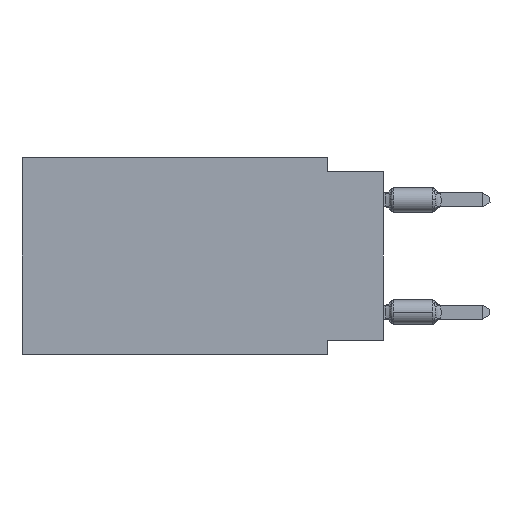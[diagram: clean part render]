
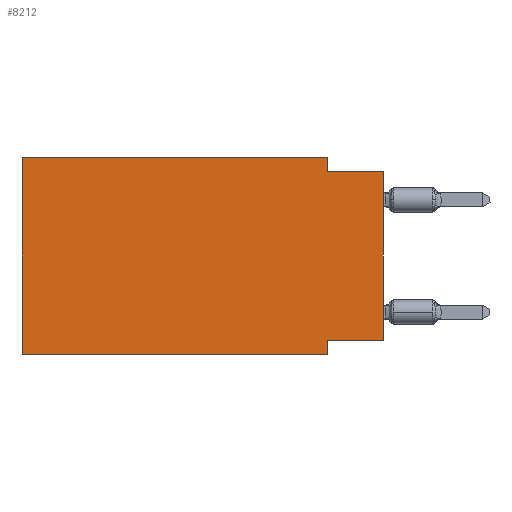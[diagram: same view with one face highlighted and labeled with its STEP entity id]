
A CAD part, left-side view. The second image highlights one B-rep face of the part: STEP entity #8212.
In plain terms, the highlighted planar face has unit normal (-1, 0, 0).
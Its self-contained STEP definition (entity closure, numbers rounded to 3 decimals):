
#36 = EDGE_CURVE ( 'NONE', #12416, #5245, #12398, .T. ) ;
#90 = DIRECTION ( 'NONE',  ( 0., -1., 0. ) ) ;
#271 = CARTESIAN_POINT ( 'NONE',  ( 0., 0., -0.635 ) ) ;
#599 = CARTESIAN_POINT ( 'NONE',  ( 0., 2.54, -0.635 ) ) ;
#840 = LINE ( 'NONE', #13821, #6699 ) ;
#1458 = DIRECTION ( 'NONE',  ( 0., -1., 0. ) ) ;
#1938 = CARTESIAN_POINT ( 'NONE',  ( 0., 0., -8.255 ) ) ;
#2111 = DIRECTION ( 'NONE',  ( 0., 1., 0. ) ) ;
#2193 = DIRECTION ( 'NONE',  ( 0., 0., 1. ) ) ;
#2235 = VERTEX_POINT ( 'NONE', #4005 ) ;
#2441 = DIRECTION ( 'NONE',  ( 0., 0., -1. ) ) ;
#2883 = ORIENTED_EDGE ( 'NONE', *, *, #16014, .F. ) ;
#3149 = CARTESIAN_POINT ( 'NONE',  ( 0., 16.383, -8.89 ) ) ;
#3205 = LINE ( 'NONE', #1938, #12406 ) ;
#3282 = VECTOR ( 'NONE', #2441, 1000. ) ;
#3781 = CARTESIAN_POINT ( 'NONE',  ( 0., 0., -8.255 ) ) ;
#3790 = EDGE_CURVE ( 'NONE', #2235, #12416, #10270, .T. ) ;
#3835 = CARTESIAN_POINT ( 'NONE',  ( 0., 2.54, -8.89 ) ) ;
#3869 = FACE_OUTER_BOUND ( 'NONE', #6715, .T. ) ;
#4005 = CARTESIAN_POINT ( 'NONE',  ( 0., 16.383, 0. ) ) ;
#4244 = CARTESIAN_POINT ( 'NONE',  ( 0., 2.54, 0. ) ) ;
#4347 = DIRECTION ( 'NONE',  ( 0., -1., 0. ) ) ;
#4388 = CARTESIAN_POINT ( 'NONE',  ( 0., 0., -0.635 ) ) ;
#5245 = VERTEX_POINT ( 'NONE', #599 ) ;
#5447 = DIRECTION ( 'NONE',  ( 0., 0., -1. ) ) ;
#5626 = LINE ( 'NONE', #3149, #8918 ) ;
#5699 = VERTEX_POINT ( 'NONE', #11560 ) ;
#6218 = VECTOR ( 'NONE', #16486, 1000. ) ;
#6660 = CARTESIAN_POINT ( 'NONE',  ( 0., 2.54, -8.255 ) ) ;
#6699 = VECTOR ( 'NONE', #2193, 1000. ) ;
#6715 = EDGE_LOOP ( 'NONE', ( #11568, #2883, #10927, #16063, #16458, #15356, #11943, #16244 ) ) ;
#7647 = EDGE_CURVE ( 'NONE', #5699, #2235, #840, .T. ) ;
#7719 = VECTOR ( 'NONE', #90, 1000. ) ;
#7919 = LINE ( 'NONE', #3835, #13597 ) ;
#8061 = AXIS2_PLACEMENT_3D ( 'NONE', #9050, #14229, #16520 ) ;
#8212 = ADVANCED_FACE ( 'NONE', ( #3869 ), #12611, .F. ) ;
#8758 = EDGE_CURVE ( 'NONE', #10169, #10735, #3205, .T. ) ;
#8918 = VECTOR ( 'NONE', #4347, 1000. ) ;
#9050 = CARTESIAN_POINT ( 'NONE',  ( 0., 16.383, 0. ) ) ;
#9596 = EDGE_CURVE ( 'NONE', #5699, #10608, #5626, .T. ) ;
#9867 = CARTESIAN_POINT ( 'NONE',  ( 0., 0., 0. ) ) ;
#10169 = VERTEX_POINT ( 'NONE', #3781 ) ;
#10270 = LINE ( 'NONE', #14008, #7719 ) ;
#10608 = VERTEX_POINT ( 'NONE', #12519 ) ;
#10735 = VERTEX_POINT ( 'NONE', #6660 ) ;
#10927 = ORIENTED_EDGE ( 'NONE', *, *, #36, .F. ) ;
#11012 = VECTOR ( 'NONE', #1458, 1000. ) ;
#11560 = CARTESIAN_POINT ( 'NONE',  ( 0., 16.383, -8.89 ) ) ;
#11568 = ORIENTED_EDGE ( 'NONE', *, *, #14661, .T. ) ;
#11943 = ORIENTED_EDGE ( 'NONE', *, *, #12275, .F. ) ;
#12275 = EDGE_CURVE ( 'NONE', #10735, #10608, #7919, .T. ) ;
#12398 = LINE ( 'NONE', #14862, #3282 ) ;
#12406 = VECTOR ( 'NONE', #2111, 1000. ) ;
#12416 = VERTEX_POINT ( 'NONE', #4244 ) ;
#12519 = CARTESIAN_POINT ( 'NONE',  ( 0., 2.54, -8.89 ) ) ;
#12611 = PLANE ( 'NONE',  #8061 ) ;
#12828 = LINE ( 'NONE', #9867, #6218 ) ;
#13086 = LINE ( 'NONE', #271, #11012 ) ;
#13597 = VECTOR ( 'NONE', #5447, 1000. ) ;
#13663 = VERTEX_POINT ( 'NONE', #4388 ) ;
#13821 = CARTESIAN_POINT ( 'NONE',  ( 0., 16.383, 0. ) ) ;
#14008 = CARTESIAN_POINT ( 'NONE',  ( 0., 16.383, 0. ) ) ;
#14229 = DIRECTION ( 'NONE',  ( 1., 0., 0. ) ) ;
#14661 = EDGE_CURVE ( 'NONE', #10169, #13663, #12828, .T. ) ;
#14862 = CARTESIAN_POINT ( 'NONE',  ( 0., 2.54, 0. ) ) ;
#15356 = ORIENTED_EDGE ( 'NONE', *, *, #9596, .T. ) ;
#16014 = EDGE_CURVE ( 'NONE', #5245, #13663, #13086, .T. ) ;
#16063 = ORIENTED_EDGE ( 'NONE', *, *, #3790, .F. ) ;
#16244 = ORIENTED_EDGE ( 'NONE', *, *, #8758, .F. ) ;
#16458 = ORIENTED_EDGE ( 'NONE', *, *, #7647, .F. ) ;
#16486 = DIRECTION ( 'NONE',  ( 0., 0., 1. ) ) ;
#16520 = DIRECTION ( 'NONE',  ( 0., 0., -1. ) ) ;
